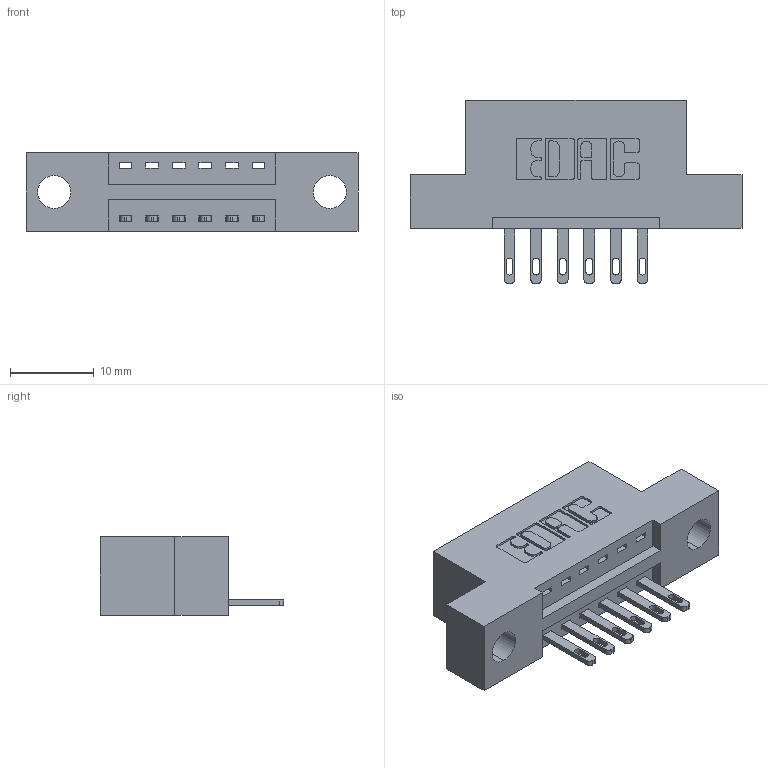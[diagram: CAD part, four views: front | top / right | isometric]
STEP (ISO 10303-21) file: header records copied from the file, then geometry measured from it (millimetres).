
FILE_DESCRIPTION (( 'STEP AP203' ), '1' );
FILE_NAME ('896-006-500-104.STEP', '2021-07-27T13:41:49', ( '' ), ( '' ), 'SwSTEP 2.0', 'SolidWorks 2020', '' );
FILE_SCHEMA (( 'CONFIG_CONTROL_DESIGN' ));
Length unit declared in the file: inch
Products named in the file (3): 896-006-500-104; 345-292-001_345-293-100; 846 Part_Flush Mounting Lugs - 0.156 Dia-TH
Assembly tree (7 placements, depth 2):
  896-006-500-104
    846 Part_Flush Mounting Lugs - 0.156 Dia-TH
    345-292-001_345-293-100  x6
Bounding box: 39.62 x 21.84 x 9.4 mm (x, y, z)
Volume: 3460.7 mm3; surface area: 3755.9 mm2
Topology: 7 solids, 7 shells, 446 faces, 1337 edges, 890 vertices
Faces by surface type: plane 280, cylinder 166
Entity records: 8503 total; most frequent: CARTESIAN_POINT 1474, ORIENTED_EDGE 1414, DIRECTION 1347, EDGE_CURVE 707, LINE 547, VECTOR 547, VERTEX_POINT 470, AXIS2_PLACEMENT_3D 400
